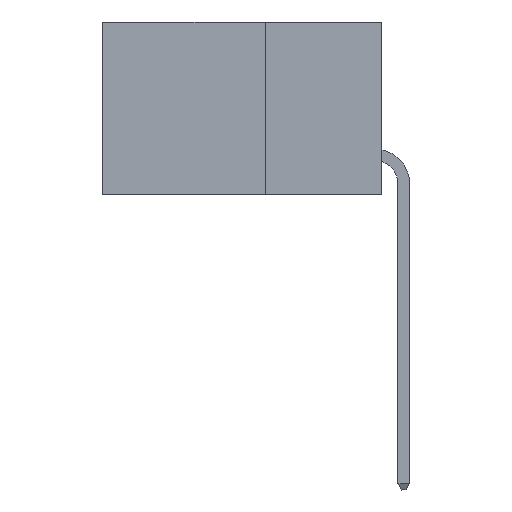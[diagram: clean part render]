
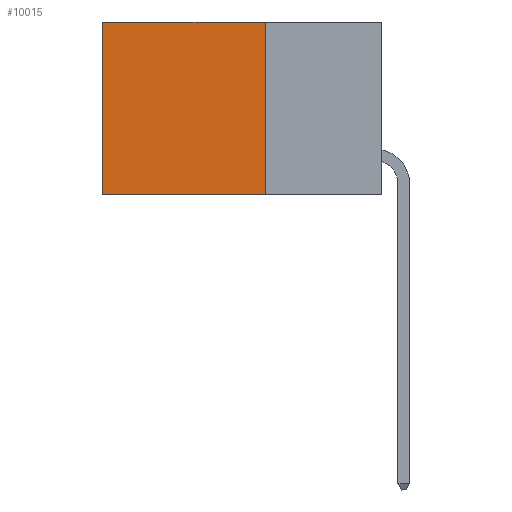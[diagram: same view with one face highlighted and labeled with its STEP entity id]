
A CAD part, left-side view. The second image highlights one B-rep face of the part: STEP entity #10015.
In plain terms, the highlighted planar face has unit normal (-1, 0, 0).
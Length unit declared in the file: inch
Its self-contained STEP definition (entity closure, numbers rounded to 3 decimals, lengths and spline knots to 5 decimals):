
#379 = VECTOR ( 'NONE', #3800, 39.37008 ) ;
#864 = PLANE ( 'NONE',  #24498 ) ;
#3550 = ORIENTED_EDGE ( 'NONE', *, *, #4648, .T. ) ;
#3800 = DIRECTION ( 'NONE',  ( 0., 1., 0. ) ) ;
#4648 = EDGE_CURVE ( 'NONE', #14837, #17051, #29399, .T. ) ;
#4903 = ORIENTED_EDGE ( 'NONE', *, *, #24915, .F. ) ;
#6117 = ORIENTED_EDGE ( 'NONE', *, *, #29788, .F. ) ;
#6315 = DIRECTION ( 'NONE',  ( 1., 0., 0. ) ) ;
#7199 = CARTESIAN_POINT ( 'NONE',  ( 0.2875, 0.6, 0. ) ) ;
#7611 = LINE ( 'NONE', #14738, #379 ) ;
#7998 = CARTESIAN_POINT ( 'NONE',  ( 0.2875, 0.25, 0. ) ) ;
#8072 = CARTESIAN_POINT ( 'NONE',  ( 0.2875, 0.6, 0. ) ) ;
#8171 = EDGE_CURVE ( 'NONE', #13321, #14837, #7611, .T. ) ;
#10015 = ADVANCED_FACE ( 'NONE', ( #10450 ), #864, .F. ) ;
#10450 = FACE_OUTER_BOUND ( 'NONE', #10881, .T. ) ;
#10881 = EDGE_LOOP ( 'NONE', ( #3550, #6117, #4903, #18038 ) ) ;
#11259 = VECTOR ( 'NONE', #21854, 39.37008 ) ;
#12979 = LINE ( 'NONE', #7998, #11259 ) ;
#13321 = VERTEX_POINT ( 'NONE', #30342 ) ;
#14738 = CARTESIAN_POINT ( 'NONE',  ( 0.2875, 0.25, 0. ) ) ;
#14837 = VERTEX_POINT ( 'NONE', #7199 ) ;
#17051 = VERTEX_POINT ( 'NONE', #18805 ) ;
#18038 = ORIENTED_EDGE ( 'NONE', *, *, #8171, .T. ) ;
#18280 = VECTOR ( 'NONE', #18945, 39.37008 ) ;
#18805 = CARTESIAN_POINT ( 'NONE',  ( 0.2875, 0.6, -0.37 ) ) ;
#18945 = DIRECTION ( 'NONE',  ( 0., 1., 0. ) ) ;
#21854 = DIRECTION ( 'NONE',  ( 0., 0., -1. ) ) ;
#22833 = CARTESIAN_POINT ( 'NONE',  ( 0.2875, 0.25, 0. ) ) ;
#24498 = AXIS2_PLACEMENT_3D ( 'NONE', #22833, #6315, #25592 ) ;
#24720 = DIRECTION ( 'NONE',  ( 0., 0., -1. ) ) ;
#24915 = EDGE_CURVE ( 'NONE', #13321, #31843, #12979, .T. ) ;
#25592 = DIRECTION ( 'NONE',  ( 0., 0., -1. ) ) ;
#25601 = LINE ( 'NONE', #27099, #18280 ) ;
#27099 = CARTESIAN_POINT ( 'NONE',  ( 0.2875, 0.25, -0.37 ) ) ;
#28543 = VECTOR ( 'NONE', #24720, 39.37008 ) ;
#29399 = LINE ( 'NONE', #8072, #28543 ) ;
#29788 = EDGE_CURVE ( 'NONE', #31843, #17051, #25601, .T. ) ;
#30014 = CARTESIAN_POINT ( 'NONE',  ( 0.2875, 0.25, -0.37 ) ) ;
#30342 = CARTESIAN_POINT ( 'NONE',  ( 0.2875, 0.25, 0. ) ) ;
#31843 = VERTEX_POINT ( 'NONE', #30014 ) ;
